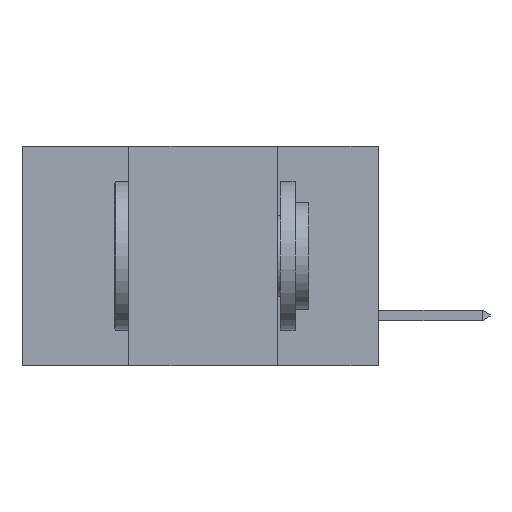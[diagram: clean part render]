
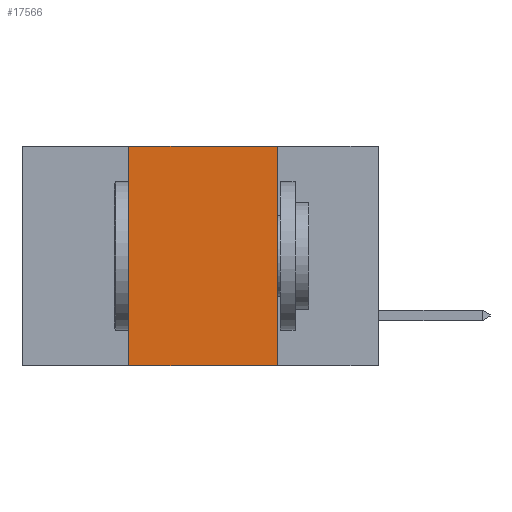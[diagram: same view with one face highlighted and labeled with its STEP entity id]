
A CAD part, left-side view. The second image highlights one B-rep face of the part: STEP entity #17566.
In plain terms, the highlighted planar face has unit normal (-1, 0, 0).
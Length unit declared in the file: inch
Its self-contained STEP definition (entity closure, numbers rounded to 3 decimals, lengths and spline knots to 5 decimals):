
#286 = LINE ( 'NONE', #9581, #1416 ) ;
#783 = EDGE_CURVE ( 'NONE', #14500, #5593, #10868, .T. ) ;
#953 = EDGE_CURVE ( 'NONE', #20868, #14500, #286, .T. ) ;
#1381 = AXIS2_PLACEMENT_3D ( 'NONE', #21046, #10141, #22820 ) ;
#1416 = VECTOR ( 'NONE', #9703, 39.37008 ) ;
#1536 = VECTOR ( 'NONE', #16116, 39.37008 ) ;
#2176 = VECTOR ( 'NONE', #19872, 39.37008 ) ;
#2733 = ORIENTED_EDGE ( 'NONE', *, *, #953, .F. ) ;
#5593 = VERTEX_POINT ( 'NONE', #10223 ) ;
#6455 = LINE ( 'NONE', #8794, #1536 ) ;
#7138 = CARTESIAN_POINT ( 'NONE',  ( 0., 0.6, -0.37 ) ) ;
#8198 = ORIENTED_EDGE ( 'NONE', *, *, #19604, .T. ) ;
#8794 = CARTESIAN_POINT ( 'NONE',  ( 0., 0.42, 0. ) ) ;
#9275 = EDGE_LOOP ( 'NONE', ( #20984, #2733, #22101, #8198 ) ) ;
#9581 = CARTESIAN_POINT ( 'NONE',  ( 0., 0.6, 0. ) ) ;
#9703 = DIRECTION ( 'NONE',  ( 0., -1., 0. ) ) ;
#10062 = PLANE ( 'NONE',  #1381 ) ;
#10141 = DIRECTION ( 'NONE',  ( 1., 0., 0. ) ) ;
#10223 = CARTESIAN_POINT ( 'NONE',  ( 0., 0.17, -0.37 ) ) ;
#10868 = LINE ( 'NONE', #23366, #22507 ) ;
#13319 = CARTESIAN_POINT ( 'NONE',  ( 0., 0.17, 0. ) ) ;
#13557 = CARTESIAN_POINT ( 'NONE',  ( 0., 0.42, -0.37 ) ) ;
#14500 = VERTEX_POINT ( 'NONE', #13319 ) ;
#14608 = CARTESIAN_POINT ( 'NONE',  ( 0., 0.42, 0. ) ) ;
#16116 = DIRECTION ( 'NONE',  ( 0., 0., 1. ) ) ;
#16210 = LINE ( 'NONE', #7138, #2176 ) ;
#17566 = ADVANCED_FACE ( 'NONE', ( #20004 ), #10062, .F. ) ;
#19347 = VERTEX_POINT ( 'NONE', #13557 ) ;
#19604 = EDGE_CURVE ( 'NONE', #19347, #5593, #16210, .T. ) ;
#19872 = DIRECTION ( 'NONE',  ( 0., -1., 0. ) ) ;
#20004 = FACE_OUTER_BOUND ( 'NONE', #9275, .T. ) ;
#20868 = VERTEX_POINT ( 'NONE', #14608 ) ;
#20984 = ORIENTED_EDGE ( 'NONE', *, *, #783, .F. ) ;
#21046 = CARTESIAN_POINT ( 'NONE',  ( 0., 0.6, 0. ) ) ;
#21537 = DIRECTION ( 'NONE',  ( 0., 0., -1. ) ) ;
#21987 = EDGE_CURVE ( 'NONE', #19347, #20868, #6455, .T. ) ;
#22101 = ORIENTED_EDGE ( 'NONE', *, *, #21987, .F. ) ;
#22507 = VECTOR ( 'NONE', #21537, 39.37008 ) ;
#22820 = DIRECTION ( 'NONE',  ( 0., 0., -1. ) ) ;
#23366 = CARTESIAN_POINT ( 'NONE',  ( 0., 0.17, 0. ) ) ;
